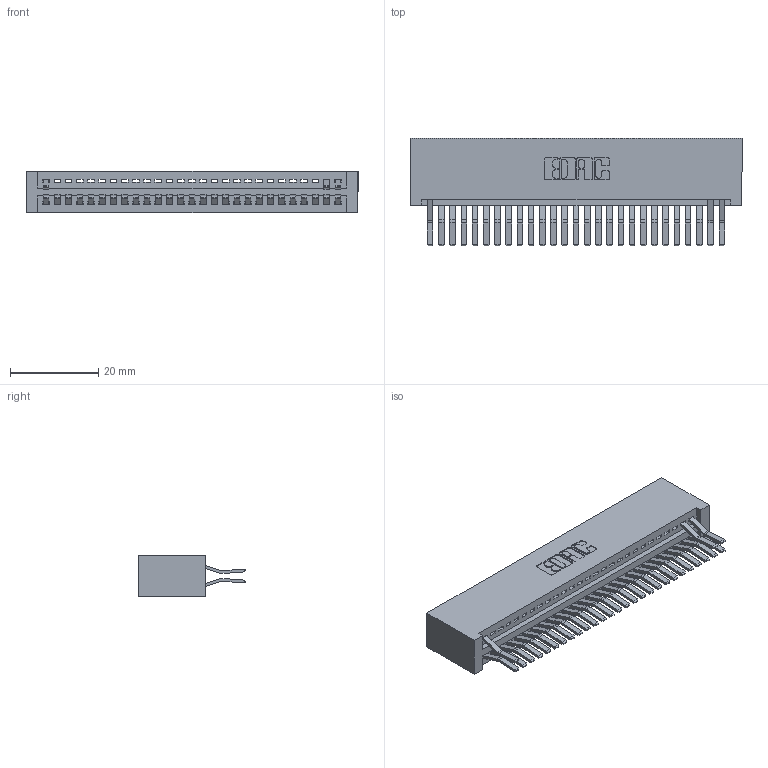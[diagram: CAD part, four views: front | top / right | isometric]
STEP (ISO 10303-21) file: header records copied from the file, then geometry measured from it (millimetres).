
FILE_DESCRIPTION (( 'STEP AP203' ), '1' );
FILE_NAME ('345-054-560-201.STEP', '2018-09-24T02:02:17', ( '' ), ( '' ), 'SwSTEP 2.0', 'SolidWorks 2016', '' );
FILE_SCHEMA (( 'CONFIG_CONTROL_DESIGN' ));
Length unit declared in the file: inch
Products named in the file (3): 345 Part_No Mounting Lugs; 345-292-001_560 Tail; 345-054-560-201
Assembly tree (31 placements, depth 2):
  345-054-560-201
    345 Part_No Mounting Lugs
    345-292-001_560 Tail  x30
Bounding box: 75.18 x 24.45 x 9.4 mm (x, y, z)
Volume: 7760.4 mm3; surface area: 10764.4 mm2
Topology: 31 solids, 31 shells, 1870 faces, 5615 edges, 3702 vertices
Faces by surface type: plane 1234, cylinder 636
Entity records: 22247 total; most frequent: CARTESIAN_POINT 3848, ORIENTED_EDGE 3806, DIRECTION 3383, EDGE_CURVE 1903, LINE 1667, VECTOR 1667, VERTEX_POINT 1266, AXIS2_PLACEMENT_3D 858
